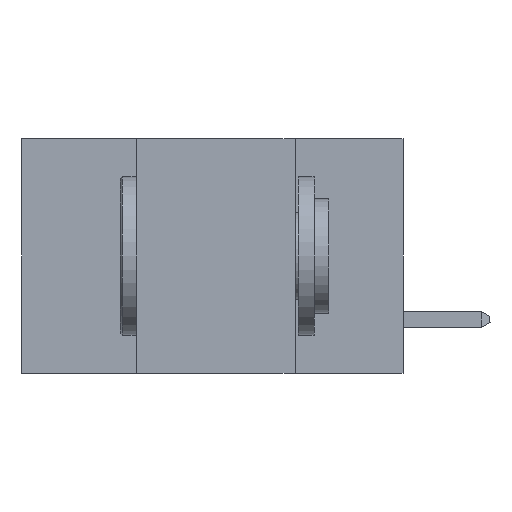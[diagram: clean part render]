
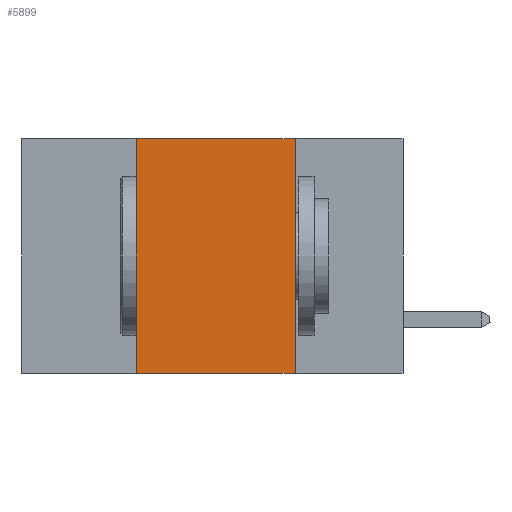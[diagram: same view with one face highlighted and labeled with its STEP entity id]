
A CAD part, left-side view. The second image highlights one B-rep face of the part: STEP entity #5899.
In plain terms, the highlighted planar face has unit normal (-1, 0, 0).
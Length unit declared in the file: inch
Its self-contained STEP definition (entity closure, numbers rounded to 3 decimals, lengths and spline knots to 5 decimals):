
#1035 = VECTOR ( 'NONE', #5513, 39.37008 ) ;
#1773 = ORIENTED_EDGE ( 'NONE', *, *, #4953, .F. ) ;
#2311 = LINE ( 'NONE', #12456, #1035 ) ;
#2518 = LINE ( 'NONE', #9643, #11275 ) ;
#3369 = VECTOR ( 'NONE', #13615, 39.37008 ) ;
#3746 = LINE ( 'NONE', #13512, #3369 ) ;
#3812 = DIRECTION ( 'NONE',  ( 1., 0., 0. ) ) ;
#3976 = FACE_OUTER_BOUND ( 'NONE', #13204, .T. ) ;
#4953 = EDGE_CURVE ( 'NONE', #11302, #13110, #2311, .T. ) ;
#5006 = CARTESIAN_POINT ( 'NONE',  ( 0., 0.6, 0. ) ) ;
#5513 = DIRECTION ( 'NONE',  ( 0., 0., 1. ) ) ;
#5899 = ADVANCED_FACE ( 'NONE', ( #3976 ), #14221, .F. ) ;
#6167 = ORIENTED_EDGE ( 'NONE', *, *, #12638, .F. ) ;
#6328 = DIRECTION ( 'NONE',  ( 0., -1., 0. ) ) ;
#6838 = VERTEX_POINT ( 'NONE', #11456 ) ;
#8026 = VERTEX_POINT ( 'NONE', #11310 ) ;
#8492 = DIRECTION ( 'NONE',  ( 0., 0., -1. ) ) ;
#9414 = ORIENTED_EDGE ( 'NONE', *, *, #14384, .T. ) ;
#9485 = DIRECTION ( 'NONE',  ( 0., -1., 0. ) ) ;
#9643 = CARTESIAN_POINT ( 'NONE',  ( 0., 0.6, -0.37 ) ) ;
#9886 = ORIENTED_EDGE ( 'NONE', *, *, #11588, .F. ) ;
#9926 = CARTESIAN_POINT ( 'NONE',  ( 0., 0.6, 0. ) ) ;
#10248 = VECTOR ( 'NONE', #6328, 39.37008 ) ;
#11275 = VECTOR ( 'NONE', #9485, 39.37008 ) ;
#11302 = VERTEX_POINT ( 'NONE', #12934 ) ;
#11310 = CARTESIAN_POINT ( 'NONE',  ( 0., 0.17, 0. ) ) ;
#11456 = CARTESIAN_POINT ( 'NONE',  ( 0., 0.17, -0.37 ) ) ;
#11588 = EDGE_CURVE ( 'NONE', #8026, #6838, #3746, .T. ) ;
#12456 = CARTESIAN_POINT ( 'NONE',  ( 0., 0.42, 0. ) ) ;
#12638 = EDGE_CURVE ( 'NONE', #13110, #8026, #14262, .T. ) ;
#12934 = CARTESIAN_POINT ( 'NONE',  ( 0., 0.42, -0.37 ) ) ;
#13110 = VERTEX_POINT ( 'NONE', #14127 ) ;
#13116 = AXIS2_PLACEMENT_3D ( 'NONE', #5006, #3812, #8492 ) ;
#13204 = EDGE_LOOP ( 'NONE', ( #9886, #6167, #1773, #9414 ) ) ;
#13512 = CARTESIAN_POINT ( 'NONE',  ( 0., 0.17, 0. ) ) ;
#13615 = DIRECTION ( 'NONE',  ( 0., 0., -1. ) ) ;
#14127 = CARTESIAN_POINT ( 'NONE',  ( 0., 0.42, 0. ) ) ;
#14221 = PLANE ( 'NONE',  #13116 ) ;
#14262 = LINE ( 'NONE', #9926, #10248 ) ;
#14384 = EDGE_CURVE ( 'NONE', #11302, #6838, #2518, .T. ) ;
